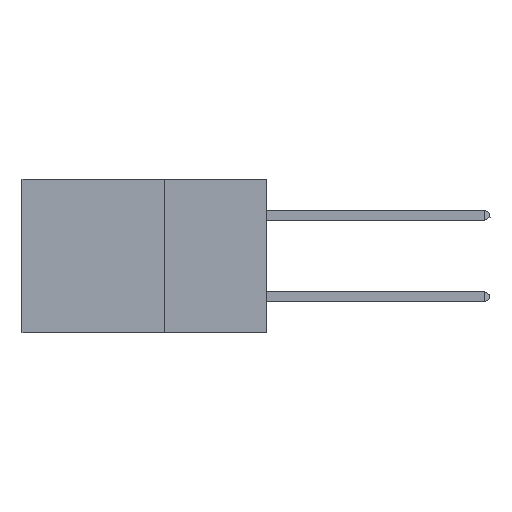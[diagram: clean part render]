
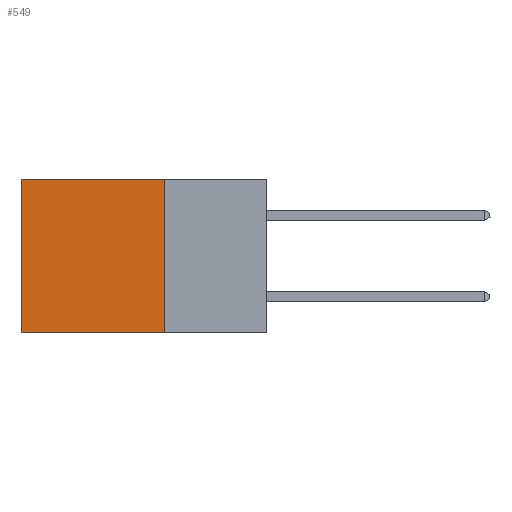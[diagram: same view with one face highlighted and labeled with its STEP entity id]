
A CAD part, left-side view. The second image highlights one B-rep face of the part: STEP entity #549.
In plain terms, the highlighted planar face has unit normal (-1, 0, 0).
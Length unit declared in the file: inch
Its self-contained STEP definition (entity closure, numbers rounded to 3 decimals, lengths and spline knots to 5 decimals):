
#146 = LINE ( 'NONE', #3605, #5581 ) ;
#153 = LINE ( 'NONE', #499, #8612 ) ;
#499 = CARTESIAN_POINT ( 'NONE',  ( 0.2875, 0.25, 0. ) ) ;
#549 = ADVANCED_FACE ( 'NONE', ( #1779 ), #8138, .F. ) ;
#1250 = VERTEX_POINT ( 'NONE', #2959 ) ;
#1295 = VERTEX_POINT ( 'NONE', #2299 ) ;
#1773 = ORIENTED_EDGE ( 'NONE', *, *, #4163, .F. ) ;
#1779 = FACE_OUTER_BOUND ( 'NONE', #6789, .T. ) ;
#2001 = ORIENTED_EDGE ( 'NONE', *, *, #2619, .F. ) ;
#2151 = DIRECTION ( 'NONE',  ( 0., 0., -1. ) ) ;
#2299 = CARTESIAN_POINT ( 'NONE',  ( 0.2875, 0.25, 0. ) ) ;
#2619 = EDGE_CURVE ( 'NONE', #4757, #8059, #146, .T. ) ;
#2890 = DIRECTION ( 'NONE',  ( 0., 1., 0. ) ) ;
#2959 = CARTESIAN_POINT ( 'NONE',  ( 0.2875, 0.6, 0. ) ) ;
#3605 = CARTESIAN_POINT ( 'NONE',  ( 0.2875, 0.25, -0.375 ) ) ;
#4163 = EDGE_CURVE ( 'NONE', #1295, #4757, #8692, .T. ) ;
#4433 = EDGE_CURVE ( 'NONE', #1250, #8059, #4843, .T. ) ;
#4446 = CARTESIAN_POINT ( 'NONE',  ( 0.2875, 0.25, -0.375 ) ) ;
#4484 = VECTOR ( 'NONE', #5542, 39.37008 ) ;
#4757 = VERTEX_POINT ( 'NONE', #8930 ) ;
#4790 = CARTESIAN_POINT ( 'NONE',  ( 0.2875, 0.25, -0.375 ) ) ;
#4842 = CARTESIAN_POINT ( 'NONE',  ( 0.2875, 0.6, -0.375 ) ) ;
#4843 = LINE ( 'NONE', #8889, #6936 ) ;
#5542 = DIRECTION ( 'NONE',  ( 0., 0., -1. ) ) ;
#5581 = VECTOR ( 'NONE', #2890, 39.37008 ) ;
#5779 = EDGE_CURVE ( 'NONE', #1295, #1250, #153, .T. ) ;
#6039 = AXIS2_PLACEMENT_3D ( 'NONE', #4446, #6724, #2151 ) ;
#6629 = DIRECTION ( 'NONE',  ( 0., 1., 0. ) ) ;
#6724 = DIRECTION ( 'NONE',  ( 1., 0., 0. ) ) ;
#6789 = EDGE_LOOP ( 'NONE', ( #7209, #2001, #1773, #7742 ) ) ;
#6936 = VECTOR ( 'NONE', #9581, 39.37008 ) ;
#7209 = ORIENTED_EDGE ( 'NONE', *, *, #4433, .T. ) ;
#7742 = ORIENTED_EDGE ( 'NONE', *, *, #5779, .T. ) ;
#8059 = VERTEX_POINT ( 'NONE', #4842 ) ;
#8138 = PLANE ( 'NONE',  #6039 ) ;
#8612 = VECTOR ( 'NONE', #6629, 39.37008 ) ;
#8692 = LINE ( 'NONE', #4790, #4484 ) ;
#8889 = CARTESIAN_POINT ( 'NONE',  ( 0.2875, 0.6, -0.375 ) ) ;
#8930 = CARTESIAN_POINT ( 'NONE',  ( 0.2875, 0.25, -0.375 ) ) ;
#9581 = DIRECTION ( 'NONE',  ( 0., 0., -1. ) ) ;
